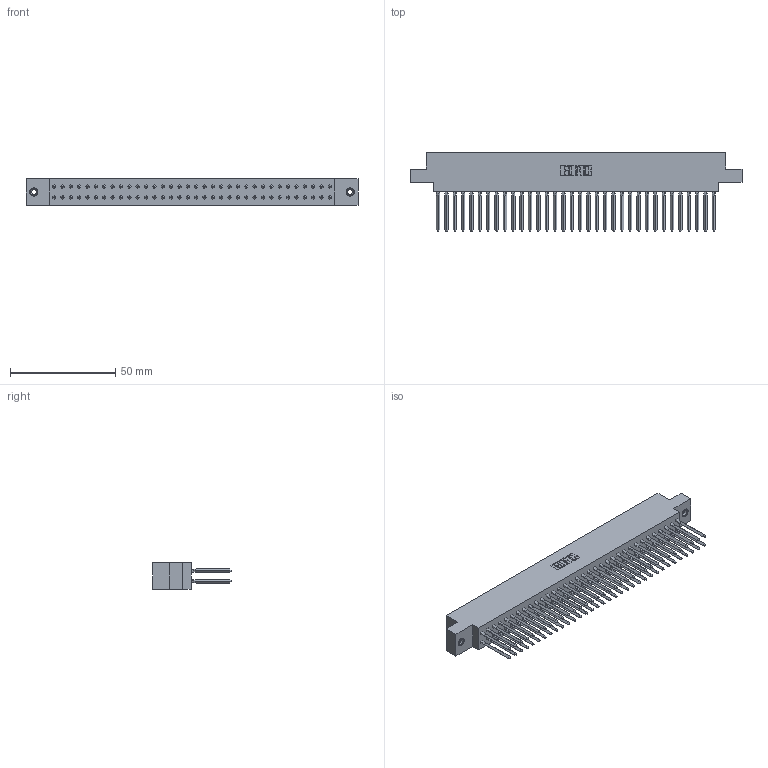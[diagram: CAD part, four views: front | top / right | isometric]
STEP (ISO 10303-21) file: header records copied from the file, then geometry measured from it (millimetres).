
FILE_DESCRIPTION (( 'STEP AP203' ), '1' );
FILE_NAME ('317-068-542-878.STEP', '2020-02-28T06:46:41', ( '' ), ( '' ), 'SwSTEP 2.0', 'SolidWorks 2016', '' );
FILE_SCHEMA (( 'CONFIG_CONTROL_DESIGN' ));
Length unit declared in the file: inch
Products named in the file (4): 317-068-542-878; 317 Part_.156 Dia - TI; 317-290-003_542; 345-250-001_345-250-003-102
Assembly tree (71 placements, depth 2):
  317-068-542-878
    317 Part_.156 Dia - TI
    317-290-003_542  x68
    345-250-001_345-250-003-102  x2
Bounding box: 157.43 x 37.34 x 12.7 mm (x, y, z)
Volume: 25519.2 mm3; surface area: 35252.6 mm2
Topology: 71 solids, 71 shells, 4038 faces, 11291 edges, 7202 vertices
Faces by surface type: plane 3218, cylinder 532, bspline 272, cone 12, torus 4
Entity records: 50466 total; most frequent: CARTESIAN_POINT 9024, ORIENTED_EDGE 8680, DIRECTION 7354, EDGE_CURVE 4340, VECTOR 4150, LINE 4150, VERTEX_POINT 2884, AXIS2_PLACEMENT_3D 1602
